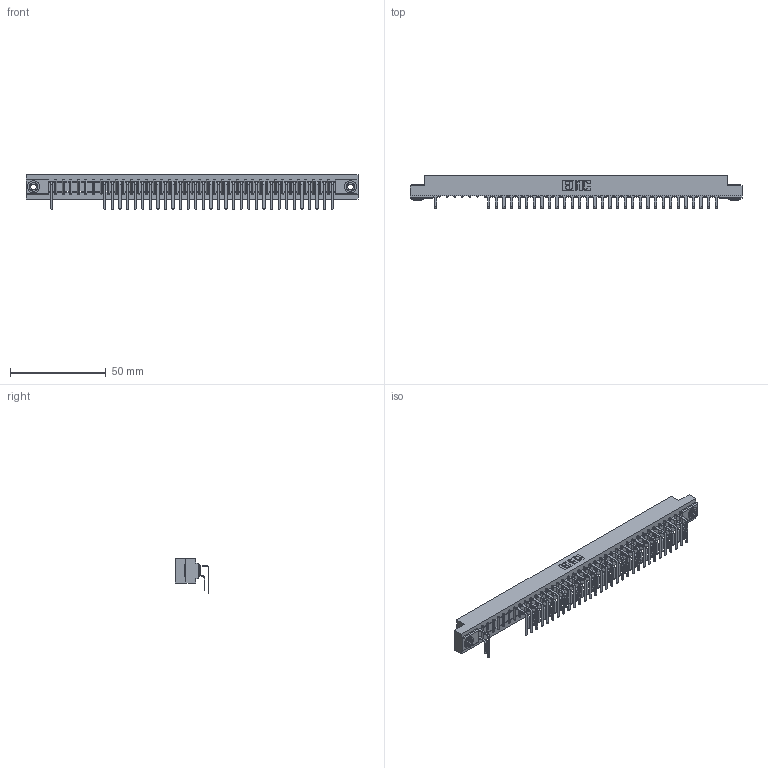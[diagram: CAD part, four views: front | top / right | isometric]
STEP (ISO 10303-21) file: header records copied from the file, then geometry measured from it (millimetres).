
FILE_DESCRIPTION (( 'STEP AP203' ), '1' );
FILE_NAME ('307-076-559-203.STEP', '2018-08-06T17:17:08', ( '' ), ( '' ), 'SwSTEP 2.0', 'SolidWorks 2016', '' );
FILE_SCHEMA (( 'CONFIG_CONTROL_DESIGN' ));
Length unit declared in the file: inch
Products named in the file (5): 345-250-002_345-250-002-102; 307-076-559-203; 307 Part_.156 Dia Mounting Holes; 307-290-001_558 559 - 1 (Single); 307-290-001_559 - 2 (Single)
Assembly tree (66 placements, depth 2):
  307-076-559-203
    307 Part_.156 Dia Mounting Holes
    307-290-001_558 559 - 1 (Single)  x31
    307-290-001_559 - 2 (Single)  x32
    345-250-002_345-250-002-102  x2
Bounding box: 173.58 x 17.69 x 18.07 mm (x, y, z)
Volume: 18544.2 mm3; surface area: 23392.2 mm2
Topology: 66 solids, 66 shells, 3489 faces, 9797 edges, 6338 vertices
Faces by surface type: plane 2251, cylinder 1152, sphere 78, cone 8
Entity records: 36382 total; most frequent: CARTESIAN_POINT 5992, ORIENTED_EDGE 5942, DIRECTION 5871, EDGE_CURVE 2971, LINE 2269, VECTOR 2269, VERTEX_POINT 1922, AXIS2_PLACEMENT_3D 1801
